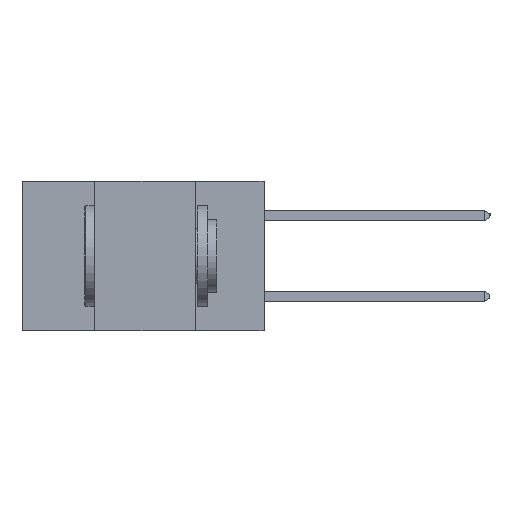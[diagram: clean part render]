
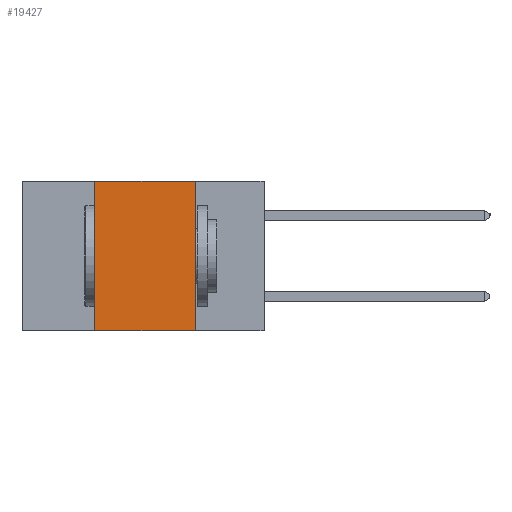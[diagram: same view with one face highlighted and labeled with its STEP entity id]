
A CAD part, left-side view. The second image highlights one B-rep face of the part: STEP entity #19427.
In plain terms, the highlighted planar face has unit normal (-1, 0, 0).
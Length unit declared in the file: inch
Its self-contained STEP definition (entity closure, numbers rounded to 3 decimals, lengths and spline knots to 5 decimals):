
#575 = CARTESIAN_POINT ( 'NONE',  ( 0., 0.6, -0.37 ) ) ;
#849 = DIRECTION ( 'NONE',  ( 0., -1., 0. ) ) ;
#996 = LINE ( 'NONE', #16381, #3582 ) ;
#1563 = ORIENTED_EDGE ( 'NONE', *, *, #5716, .T. ) ;
#2907 = DIRECTION ( 'NONE',  ( 0., 0., -1. ) ) ;
#2948 = CARTESIAN_POINT ( 'NONE',  ( 0., 0.6, 0. ) ) ;
#3142 = LINE ( 'NONE', #575, #13114 ) ;
#3328 = CARTESIAN_POINT ( 'NONE',  ( 0., 0.17, -0.37 ) ) ;
#3582 = VECTOR ( 'NONE', #849, 39.37008 ) ;
#5113 = FACE_OUTER_BOUND ( 'NONE', #20518, .T. ) ;
#5716 = EDGE_CURVE ( 'NONE', #24919, #18959, #3142, .T. ) ;
#6655 = EDGE_CURVE ( 'NONE', #24919, #26142, #11837, .T. ) ;
#8000 = AXIS2_PLACEMENT_3D ( 'NONE', #2948, #11738, #18353 ) ;
#9377 = CARTESIAN_POINT ( 'NONE',  ( 0., 0.42, -0.37 ) ) ;
#9944 = DIRECTION ( 'NONE',  ( 0., 0., 1. ) ) ;
#11738 = DIRECTION ( 'NONE',  ( 1., 0., 0. ) ) ;
#11837 = LINE ( 'NONE', #9377, #25029 ) ;
#13114 = VECTOR ( 'NONE', #17993, 39.37008 ) ;
#13380 = CARTESIAN_POINT ( 'NONE',  ( 0., 0.17, -0.37 ) ) ;
#14644 = ORIENTED_EDGE ( 'NONE', *, *, #6655, .F. ) ;
#15037 = VECTOR ( 'NONE', #2907, 39.37008 ) ;
#15782 = CARTESIAN_POINT ( 'NONE',  ( 0., 0.17, 0. ) ) ;
#16381 = CARTESIAN_POINT ( 'NONE',  ( 0., 0.6, 0. ) ) ;
#16494 = ORIENTED_EDGE ( 'NONE', *, *, #24897, .F. ) ;
#17993 = DIRECTION ( 'NONE',  ( 0., -1., 0. ) ) ;
#18353 = DIRECTION ( 'NONE',  ( 0., 0., -1. ) ) ;
#18849 = ORIENTED_EDGE ( 'NONE', *, *, #28301, .F. ) ;
#18959 = VERTEX_POINT ( 'NONE', #13380 ) ;
#19427 = ADVANCED_FACE ( 'NONE', ( #5113 ), #22631, .F. ) ;
#19788 = CARTESIAN_POINT ( 'NONE',  ( 0., 0.42, 0. ) ) ;
#20518 = EDGE_LOOP ( 'NONE', ( #16494, #18849, #14644, #1563 ) ) ;
#20870 = CARTESIAN_POINT ( 'NONE',  ( 0., 0.42, -0.37 ) ) ;
#21009 = LINE ( 'NONE', #3328, #15037 ) ;
#22457 = VERTEX_POINT ( 'NONE', #15782 ) ;
#22631 = PLANE ( 'NONE',  #8000 ) ;
#24897 = EDGE_CURVE ( 'NONE', #22457, #18959, #21009, .T. ) ;
#24919 = VERTEX_POINT ( 'NONE', #20870 ) ;
#25029 = VECTOR ( 'NONE', #9944, 39.37008 ) ;
#26142 = VERTEX_POINT ( 'NONE', #19788 ) ;
#28301 = EDGE_CURVE ( 'NONE', #26142, #22457, #996, .T. ) ;
